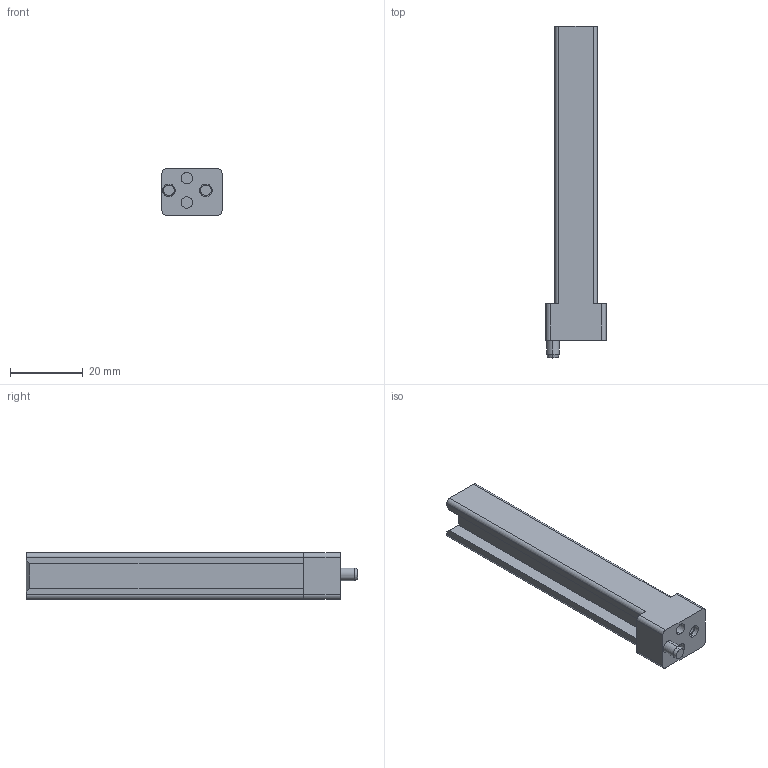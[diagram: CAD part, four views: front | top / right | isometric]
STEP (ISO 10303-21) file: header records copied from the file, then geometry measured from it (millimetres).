
FILE_DESCRIPTION (( 'STEP AP214' ), '1' );
FILE_NAME ('243-220-302.STEP', '2020-08-19T15:27:40', ( '' ), ( '' ), 'SwSTEP 2.0', 'SolidWorks 2020', '' );
FILE_SCHEMA (( 'AUTOMOTIVE_DESIGN' ));
Length unit declared in the file: inch
Products named in the file (1): 243-220-302
Bounding box: 16.51 x 91.19 x 12.7 mm (x, y, z)
Volume: 9457.5 mm3; surface area: 5948.8 mm2
Topology: 1 solids, 1 shells, 179 faces, 462 edges, 306 vertices
Faces by surface type: plane 127, bspline 32, cylinder 18, cone 2
Entity records: 7294 total; most frequent: CARTESIAN_POINT 3060, ORIENTED_EDGE 924, DIRECTION 732, EDGE_CURVE 462, LINE 360, VECTOR 360, VERTEX_POINT 306, EDGE_LOOP 200
